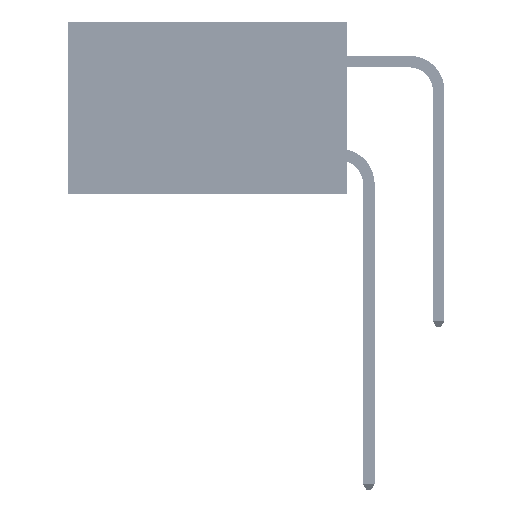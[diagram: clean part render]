
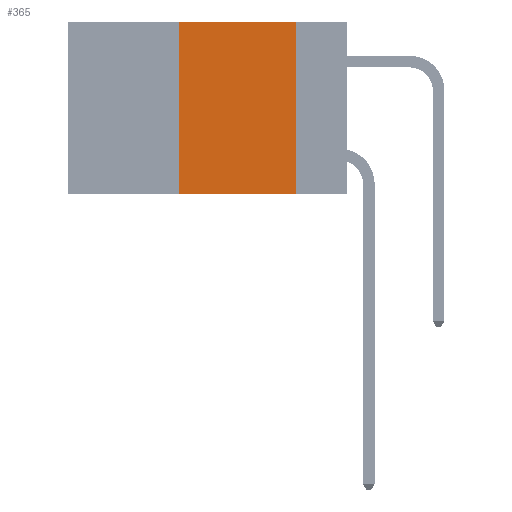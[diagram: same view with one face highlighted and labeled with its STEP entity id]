
A CAD part, left-side view. The second image highlights one B-rep face of the part: STEP entity #365.
In plain terms, the highlighted planar face has unit normal (-1, 0, 0).
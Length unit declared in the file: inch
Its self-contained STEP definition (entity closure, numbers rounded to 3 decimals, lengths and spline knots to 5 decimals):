
#365 = ADVANCED_FACE ( 'NONE', ( #24668 ), #25249, .F. ) ;
#1879 = VERTEX_POINT ( 'NONE', #50923 ) ;
#2033 = DIRECTION ( 'NONE',  ( 0., -1., 0. ) ) ;
#2522 = LINE ( 'NONE', #3304, #5176 ) ;
#3304 = CARTESIAN_POINT ( 'NONE',  ( 0., 0.36, 0. ) ) ;
#5176 = VECTOR ( 'NONE', #37023, 39.37008 ) ;
#5925 = CARTESIAN_POINT ( 'NONE',  ( 0., 0.6, -0.37 ) ) ;
#7822 = CARTESIAN_POINT ( 'NONE',  ( 0., 0.6, 0. ) ) ;
#14174 = ORIENTED_EDGE ( 'NONE', *, *, #21907, .F. ) ;
#15828 = LINE ( 'NONE', #5925, #44315 ) ;
#16162 = VECTOR ( 'NONE', #47418, 39.37008 ) ;
#21907 = EDGE_CURVE ( 'NONE', #41404, #51784, #54538, .T. ) ;
#22540 = ORIENTED_EDGE ( 'NONE', *, *, #44327, .T. ) ;
#22799 = AXIS2_PLACEMENT_3D ( 'NONE', #7822, #33036, #37289 ) ;
#24668 = FACE_OUTER_BOUND ( 'NONE', #38534, .T. ) ;
#25249 = PLANE ( 'NONE',  #22799 ) ;
#25399 = EDGE_CURVE ( 'NONE', #50478, #41404, #45615, .T. ) ;
#26137 = CARTESIAN_POINT ( 'NONE',  ( 0., 0.11, 0. ) ) ;
#29031 = VECTOR ( 'NONE', #29479, 39.37008 ) ;
#29479 = DIRECTION ( 'NONE',  ( 0., -1., 0. ) ) ;
#32472 = ORIENTED_EDGE ( 'NONE', *, *, #25399, .F. ) ;
#33036 = DIRECTION ( 'NONE',  ( 1., 0., 0. ) ) ;
#33479 = CARTESIAN_POINT ( 'NONE',  ( 0., 0.36, 0. ) ) ;
#37023 = DIRECTION ( 'NONE',  ( 0., 0., 1. ) ) ;
#37289 = DIRECTION ( 'NONE',  ( 0., 0., -1. ) ) ;
#38534 = EDGE_LOOP ( 'NONE', ( #14174, #32472, #39533, #22540 ) ) ;
#39533 = ORIENTED_EDGE ( 'NONE', *, *, #44559, .F. ) ;
#41404 = VERTEX_POINT ( 'NONE', #50338 ) ;
#44315 = VECTOR ( 'NONE', #2033, 39.37008 ) ;
#44327 = EDGE_CURVE ( 'NONE', #1879, #51784, #15828, .T. ) ;
#44559 = EDGE_CURVE ( 'NONE', #1879, #50478, #2522, .T. ) ;
#45615 = LINE ( 'NONE', #54782, #29031 ) ;
#46899 = CARTESIAN_POINT ( 'NONE',  ( 0., 0.11, -0.37 ) ) ;
#47418 = DIRECTION ( 'NONE',  ( 0., 0., -1. ) ) ;
#50338 = CARTESIAN_POINT ( 'NONE',  ( 0., 0.11, 0. ) ) ;
#50478 = VERTEX_POINT ( 'NONE', #33479 ) ;
#50923 = CARTESIAN_POINT ( 'NONE',  ( 0., 0.36, -0.37 ) ) ;
#51784 = VERTEX_POINT ( 'NONE', #46899 ) ;
#54538 = LINE ( 'NONE', #26137, #16162 ) ;
#54782 = CARTESIAN_POINT ( 'NONE',  ( 0., 0.6, 0. ) ) ;
